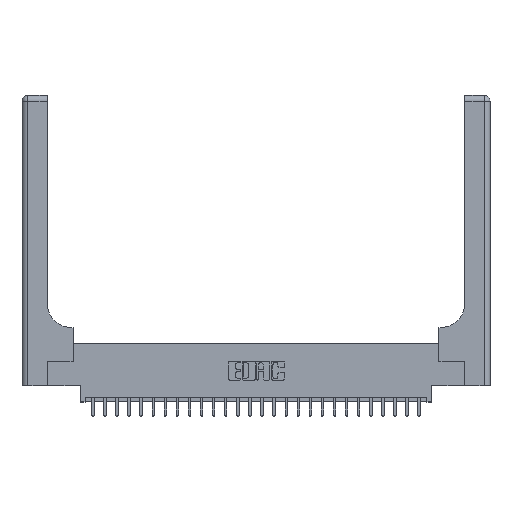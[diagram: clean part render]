
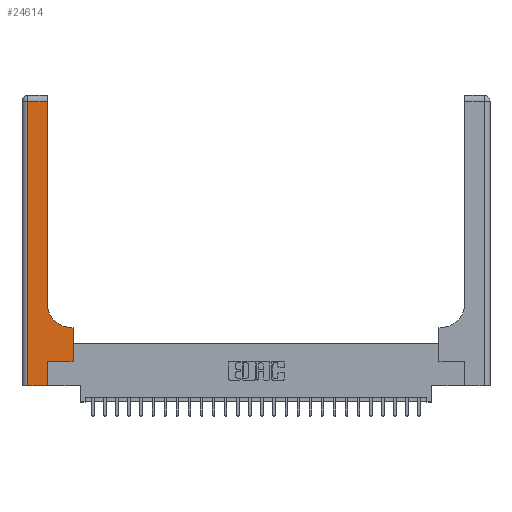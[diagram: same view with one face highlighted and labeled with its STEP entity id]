
A CAD part, top view. The second image highlights one B-rep face of the part: STEP entity #24614.
In plain terms, the highlighted planar face has unit normal (0, 0, 1).
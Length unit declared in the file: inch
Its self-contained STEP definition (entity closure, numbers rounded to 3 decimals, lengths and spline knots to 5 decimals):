
#483 = CARTESIAN_POINT ( 'NONE',  ( 0.06, 3., 0.37 ) ) ;
#541 = CARTESIAN_POINT ( 'NONE',  ( 0.51, 0.6, 0.37 ) ) ;
#916 = CARTESIAN_POINT ( 'NONE',  ( 0.26, 3., 0.37 ) ) ;
#1342 = ORIENTED_EDGE ( 'NONE', *, *, #14091, .T. ) ;
#1988 = ORIENTED_EDGE ( 'NONE', *, *, #12142, .T. ) ;
#2944 = EDGE_CURVE ( 'NONE', #3603, #11404, #16087, .T. ) ;
#3058 = VERTEX_POINT ( 'NONE', #541 ) ;
#3603 = VERTEX_POINT ( 'NONE', #16027 ) ;
#3615 = DIRECTION ( 'NONE',  ( -1., 0., 0. ) ) ;
#4207 = EDGE_CURVE ( 'NONE', #11176, #5193, #23533, .T. ) ;
#4351 = CARTESIAN_POINT ( 'NONE',  ( 0.265, 0.25, 0.37 ) ) ;
#4391 = LINE ( 'NONE', #12578, #15979 ) ;
#4762 = CARTESIAN_POINT ( 'NONE',  ( 0.06, 2.94, 0.37 ) ) ;
#4927 = ORIENTED_EDGE ( 'NONE', *, *, #8178, .T. ) ;
#5134 = VERTEX_POINT ( 'NONE', #10427 ) ;
#5193 = VERTEX_POINT ( 'NONE', #4351 ) ;
#5282 = EDGE_LOOP ( 'NONE', ( #23018, #18284, #5989, #5982, #18756, #4927, #1988, #1342, #15133 ) ) ;
#5333 = VECTOR ( 'NONE', #18395, 39.37008 ) ;
#5501 = LINE ( 'NONE', #11443, #18521 ) ;
#5596 = PLANE ( 'NONE',  #17586 ) ;
#5790 = VECTOR ( 'NONE', #17680, 39.37008 ) ;
#5849 = CARTESIAN_POINT ( 'NONE',  ( 0., 3., 0.37 ) ) ;
#5946 = CARTESIAN_POINT ( 'NONE',  ( 0., 0., 0.37 ) ) ;
#5967 = EDGE_CURVE ( 'NONE', #11404, #15471, #10724, .T. ) ;
#5982 = ORIENTED_EDGE ( 'NONE', *, *, #16439, .T. ) ;
#5989 = ORIENTED_EDGE ( 'NONE', *, *, #5967, .T. ) ;
#6141 = EDGE_CURVE ( 'NONE', #3058, #24459, #13473, .T. ) ;
#6427 = LINE ( 'NONE', #18384, #22147 ) ;
#6696 = VECTOR ( 'NONE', #8732, 39.37008 ) ;
#7088 = DIRECTION ( 'NONE',  ( -1., 0., 0. ) ) ;
#8178 = EDGE_CURVE ( 'NONE', #5193, #5134, #4391, .T. ) ;
#8732 = DIRECTION ( 'NONE',  ( 0., -1., 0. ) ) ;
#8912 = LINE ( 'NONE', #916, #14192 ) ;
#9149 = CARTESIAN_POINT ( 'NONE',  ( 0.26, 0.85, 0.37 ) ) ;
#9273 = DIRECTION ( 'NONE',  ( 1., 0., 0. ) ) ;
#9781 = CARTESIAN_POINT ( 'NONE',  ( 0.528, 0.6, 0.37 ) ) ;
#9909 = VERTEX_POINT ( 'NONE', #9781 ) ;
#10394 = CARTESIAN_POINT ( 'NONE',  ( 0., 2.94, 0.37 ) ) ;
#10427 = CARTESIAN_POINT ( 'NONE',  ( 0.528, 0.25, 0.37 ) ) ;
#10724 = LINE ( 'NONE', #483, #6696 ) ;
#11176 = VERTEX_POINT ( 'NONE', #23987 ) ;
#11404 = VERTEX_POINT ( 'NONE', #4762 ) ;
#11443 = CARTESIAN_POINT ( 'NONE',  ( 0.26, 0.6, 0.37 ) ) ;
#12050 = FACE_OUTER_BOUND ( 'NONE', #5282, .T. ) ;
#12142 = EDGE_CURVE ( 'NONE', #5134, #9909, #6427, .T. ) ;
#12578 = CARTESIAN_POINT ( 'NONE',  ( 0.265, 0.25, 0.37 ) ) ;
#13473 = CIRCLE ( 'NONE', #23517, 0.25 ) ;
#14091 = EDGE_CURVE ( 'NONE', #9909, #3058, #5501, .T. ) ;
#14192 = VECTOR ( 'NONE', #17476, 39.37008 ) ;
#15133 = ORIENTED_EDGE ( 'NONE', *, *, #6141, .T. ) ;
#15444 = CARTESIAN_POINT ( 'NONE',  ( 0.06, 0., 0.37 ) ) ;
#15471 = VERTEX_POINT ( 'NONE', #15444 ) ;
#15979 = VECTOR ( 'NONE', #22543, 39.37008 ) ;
#16027 = CARTESIAN_POINT ( 'NONE',  ( 0.26, 2.94, 0.37 ) ) ;
#16087 = LINE ( 'NONE', #10394, #5333 ) ;
#16344 = VECTOR ( 'NONE', #17671, 39.37008 ) ;
#16439 = EDGE_CURVE ( 'NONE', #15471, #11176, #23832, .T. ) ;
#17431 = DIRECTION ( 'NONE',  ( 0., 0., -1. ) ) ;
#17476 = DIRECTION ( 'NONE',  ( 0., 1., 0. ) ) ;
#17586 = AXIS2_PLACEMENT_3D ( 'NONE', #5849, #20023, #3615 ) ;
#17671 = DIRECTION ( 'NONE',  ( 1., 0., 0. ) ) ;
#17680 = DIRECTION ( 'NONE',  ( 0., 1., 0. ) ) ;
#17801 = CARTESIAN_POINT ( 'NONE',  ( 0.265, 0., 0.37 ) ) ;
#18284 = ORIENTED_EDGE ( 'NONE', *, *, #2944, .T. ) ;
#18384 = CARTESIAN_POINT ( 'NONE',  ( 0.528, 0.25, 0.37 ) ) ;
#18395 = DIRECTION ( 'NONE',  ( -1., 0., 0. ) ) ;
#18521 = VECTOR ( 'NONE', #7088, 39.37008 ) ;
#18756 = ORIENTED_EDGE ( 'NONE', *, *, #4207, .T. ) ;
#20023 = DIRECTION ( 'NONE',  ( 0., 0., -1. ) ) ;
#22147 = VECTOR ( 'NONE', #24178, 39.37008 ) ;
#22543 = DIRECTION ( 'NONE',  ( 1., 0., 0. ) ) ;
#22752 = EDGE_CURVE ( 'NONE', #24459, #3603, #8912, .T. ) ;
#23018 = ORIENTED_EDGE ( 'NONE', *, *, #22752, .T. ) ;
#23339 = CARTESIAN_POINT ( 'NONE',  ( 0.51, 0.85, 0.37 ) ) ;
#23517 = AXIS2_PLACEMENT_3D ( 'NONE', #23339, #17431, #9273 ) ;
#23533 = LINE ( 'NONE', #17801, #5790 ) ;
#23832 = LINE ( 'NONE', #5946, #16344 ) ;
#23987 = CARTESIAN_POINT ( 'NONE',  ( 0.265, 0., 0.37 ) ) ;
#24178 = DIRECTION ( 'NONE',  ( 0., 1., 0. ) ) ;
#24459 = VERTEX_POINT ( 'NONE', #9149 ) ;
#24614 = ADVANCED_FACE ( 'NONE', ( #12050 ), #5596, .F. ) ;
